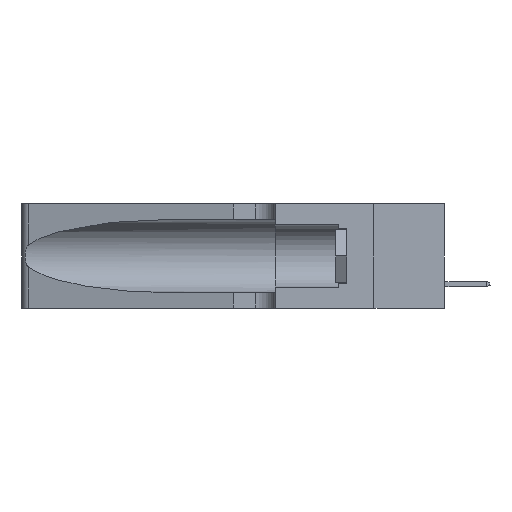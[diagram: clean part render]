
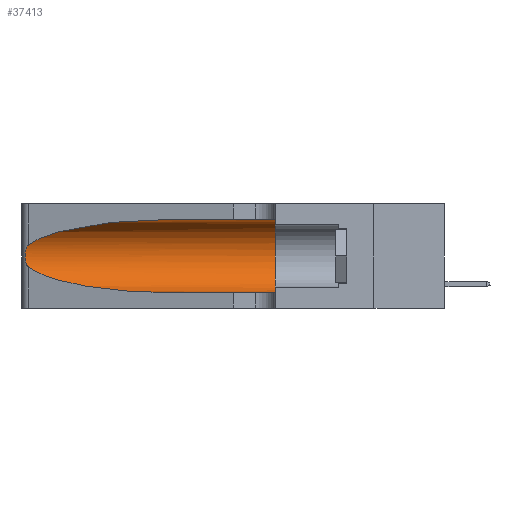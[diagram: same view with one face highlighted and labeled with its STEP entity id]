
A CAD part, left-side view. The second image highlights one B-rep face of the part: STEP entity #37413.
In plain terms, the highlighted cylindrical face has radius 3.308 mm (diameter 6.617 mm), a partial arc.
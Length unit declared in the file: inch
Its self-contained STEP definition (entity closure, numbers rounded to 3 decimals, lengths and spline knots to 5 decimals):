
#112 = CARTESIAN_POINT ( 'NONE',  ( 0.25487, 1.22718, 0.22369 ) ) ;
#835 = VERTEX_POINT ( 'NONE', #26656 ) ;
#910 = VERTEX_POINT ( 'NONE', #9639 ) ;
#1004 = ORIENTED_EDGE ( 'NONE', *, *, #39473, .T. ) ;
#1789 = CARTESIAN_POINT ( 'NONE',  ( 0.1305, 0.72297, 0.05475 ) ) ;
#3613 = CARTESIAN_POINT ( 'NONE',  ( 0.1305, 1.61858, 0.05475 ) ) ;
#4595 = VERTEX_POINT ( 'NONE', #5126 ) ;
#4980 = CARTESIAN_POINT ( 'NONE',  ( 0.25854, 1.2359, 0.20912 ) ) ;
#4989 = CARTESIAN_POINT ( 'NONE',  ( 0.25487, 1.22718, 0.14631 ) ) ;
#5126 = CARTESIAN_POINT ( 'NONE',  ( 0.1305, 0.35, 0.05475 ) ) ;
#6794 = CARTESIAN_POINT ( 'NONE',  ( 0.1305, 1.61858, 0.185 ) ) ;
#6850 = DIRECTION ( 'NONE',  ( 0., 1., 0. ) ) ;
#6967 = CIRCLE ( 'NONE', #18002, 0.13025 ) ;
#7280 = CARTESIAN_POINT ( 'NONE',  ( 0.2373, 1.15595, 0.28018 ) ) ;
#7854 = VECTOR ( 'NONE', #8394, 39.37008 ) ;
#8394 = DIRECTION ( 'NONE',  ( 0., -1., 0. ) ) ;
#9639 = CARTESIAN_POINT ( 'NONE',  ( 0.1305, 0.72297, 0.31525 ) ) ;
#9881 = DIRECTION ( 'NONE',  ( 0., 0., -1. ) ) ;
#10183 = DIRECTION ( 'NONE',  ( 0., 0., 1. ) ) ;
#10441 = ORIENTED_EDGE ( 'NONE', *, *, #38631, .F. ) ;
#10485 = CARTESIAN_POINT ( 'NONE',  ( 0.25639, 1.23186, 0.15144 ) ) ;
#11440 = EDGE_LOOP ( 'NONE', ( #30264, #31780, #1004, #20024, #10441, #28054 ) ) ;
#12621 = CARTESIAN_POINT ( 'NONE',  ( 0.25555, 1.22994, 0.2215 ) ) ;
#13541 = CARTESIAN_POINT ( 'NONE',  ( 0.25555, 1.22993, 0.14849 ) ) ;
#13822 = LINE ( 'NONE', #3613, #30816 ) ;
#14553 = EDGE_CURVE ( 'NONE', #835, #20728, #36204, .T. ) ;
#14603 =( BOUNDED_CURVE ( )  B_SPLINE_CURVE ( 3, ( #35804, #32836, #23637, #1789 ),
 .UNSPECIFIED., .F., .F. ) 
 B_SPLINE_CURVE_WITH_KNOTS ( ( 4, 4 ),
 ( 3.44316, 4.71239 ),
 .UNSPECIFIED. ) 
 CURVE ( )  GEOMETRIC_REPRESENTATION_ITEM ( )  RATIONAL_B_SPLINE_CURVE ( ( 1., 0.87, 0.87, 1. ) ) 
 REPRESENTATION_ITEM ( '' )  );
#16968 = CARTESIAN_POINT ( 'NONE',  ( 0.1305, 0.72297, 0.31525 ) ) ;
#17001 = CARTESIAN_POINT ( 'NONE',  ( 0.1305, 1.61858, 0.31525 ) ) ;
#17109 = CARTESIAN_POINT ( 'NONE',  ( 0.26017, 1.23833, 0.17102 ) ) ;
#18002 = AXIS2_PLACEMENT_3D ( 'NONE', #28443, #6850, #10183 ) ;
#19026 = DIRECTION ( 'NONE',  ( 0., -1., 0. ) ) ;
#20024 = ORIENTED_EDGE ( 'NONE', *, *, #29769, .T. ) ;
#20108 = FACE_OUTER_BOUND ( 'NONE', #11440, .T. ) ;
#20728 = VERTEX_POINT ( 'NONE', #4989 ) ;
#21364 = LINE ( 'NONE', #17001, #7854 ) ;
#22634 = EDGE_CURVE ( 'NONE', #910, #31533, #21364, .T. ) ;
#23158 = CARTESIAN_POINT ( 'NONE',  ( 0.1305, 0.35, 0.31525 ) ) ;
#23637 = CARTESIAN_POINT ( 'NONE',  ( 0.18966, 0.96281, 0.05475 ) ) ;
#25210 = VERTEX_POINT ( 'NONE', #29486 ) ;
#25746 = AXIS2_PLACEMENT_3D ( 'NONE', #6794, #19026, #9881 ) ;
#26656 = CARTESIAN_POINT ( 'NONE',  ( 0.25487, 1.22718, 0.22369 ) ) ;
#28054 = ORIENTED_EDGE ( 'NONE', *, *, #22634, .F. ) ;
#28443 = CARTESIAN_POINT ( 'NONE',  ( 0.1305, 0.35, 0.185 ) ) ;
#28574 = DIRECTION ( 'NONE',  ( 0., -1., 0. ) ) ;
#29486 = CARTESIAN_POINT ( 'NONE',  ( 0.1305, 0.72297, 0.05475 ) ) ;
#29553 = CARTESIAN_POINT ( 'NONE',  ( 0.25789, 1.23486, 0.15765 ) ) ;
#29769 = EDGE_CURVE ( 'NONE', #25210, #4595, #13822, .T. ) ;
#30264 = ORIENTED_EDGE ( 'NONE', *, *, #38111, .T. ) ;
#30816 = VECTOR ( 'NONE', #28574, 39.37008 ) ;
#31533 = VERTEX_POINT ( 'NONE', #23158 ) ;
#31780 = ORIENTED_EDGE ( 'NONE', *, *, #14553, .T. ) ;
#32836 = CARTESIAN_POINT ( 'NONE',  ( 0.2373, 1.15595, 0.08982 ) ) ;
#35103 = CARTESIAN_POINT ( 'NONE',  ( 0.18966, 0.96281, 0.31525 ) ) ;
#35224 = CARTESIAN_POINT ( 'NONE',  ( 0.25856, 1.23593, 0.16098 ) ) ;
#35348 = CARTESIAN_POINT ( 'NONE',  ( 0.26075, 1.23896, 0.19203 ) ) ;
#35614 = CARTESIAN_POINT ( 'NONE',  ( 0.25787, 1.23484, 0.2124 ) ) ;
#35804 = CARTESIAN_POINT ( 'NONE',  ( 0.25487, 1.22718, 0.14631 ) ) ;
#35882 = CARTESIAN_POINT ( 'NONE',  ( 0.25487, 1.22718, 0.14631 ) ) ;
#36204 = B_SPLINE_CURVE_WITH_KNOTS ( 'NONE', 3,
 ( #112, #12621, #38864, #35614, #4980, #38310, #35348, #38586, #17109, #35224, #29553, #10485, #13541, #35882 ),
 .UNSPECIFIED., .F., .F.,
 ( 4, 2, 2, 2, 2, 2, 4 ),
 ( 0., 0.00027, 0.00053, 0.00107, 0.0016, 0.00187, 0.00214 ),
 .UNSPECIFIED. ) ;
#37413 = ADVANCED_FACE ( 'NONE', ( #20108 ), #37986, .F. ) ;
#37986 = CYLINDRICAL_SURFACE ( 'NONE', #25746, 0.13025 ) ;
#38111 = EDGE_CURVE ( 'NONE', #910, #835, #38141, .T. ) ;
#38141 =( BOUNDED_CURVE ( )  B_SPLINE_CURVE ( 3, ( #16968, #35103, #7280, #38606 ),
 .UNSPECIFIED., .F., .F. ) 
 B_SPLINE_CURVE_WITH_KNOTS ( ( 4, 4 ),
 ( 1.5708, 2.84003 ),
 .UNSPECIFIED. ) 
 CURVE ( )  GEOMETRIC_REPRESENTATION_ITEM ( )  RATIONAL_B_SPLINE_CURVE ( ( 1., 0.87, 0.87, 1. ) ) 
 REPRESENTATION_ITEM ( '' )  );
#38310 = CARTESIAN_POINT ( 'NONE',  ( 0.26018, 1.23835, 0.19895 ) ) ;
#38586 = CARTESIAN_POINT ( 'NONE',  ( 0.26075, 1.23896, 0.178 ) ) ;
#38606 = CARTESIAN_POINT ( 'NONE',  ( 0.25487, 1.22718, 0.22369 ) ) ;
#38631 = EDGE_CURVE ( 'NONE', #31533, #4595, #6967, .T. ) ;
#38864 = CARTESIAN_POINT ( 'NONE',  ( 0.25639, 1.23184, 0.21858 ) ) ;
#39473 = EDGE_CURVE ( 'NONE', #20728, #25210, #14603, .T. ) ;
